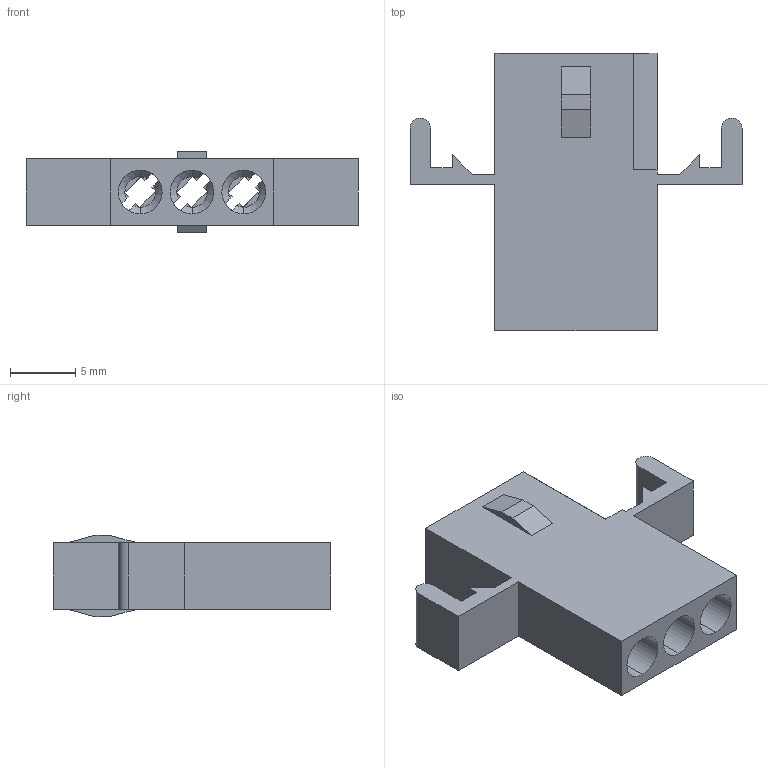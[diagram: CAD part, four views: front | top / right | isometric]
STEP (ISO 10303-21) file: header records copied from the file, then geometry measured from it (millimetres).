
FILE_DESCRIPTION (( 'STEP AP203' ), '1' );
FILE_NAME ('556-003-000-102.STEP', '2020-03-13T14:18:30', ( '' ), ( '' ), 'SwSTEP 2.0', 'SolidWorks 2016', '' );
FILE_SCHEMA (( 'CONFIG_CONTROL_DESIGN' ));
Length unit declared in the file: millimetre
Products named in the file (2): 556-003-000-102; 556-210-001_556-003-000-102
Assembly tree (1 placements, depth 2):
  556-003-000-102
    556-210-001_556-003-000-102
Bounding box: 25.4 x 21.21 x 6.22 mm (x, y, z)
Volume: 992.5 mm3; surface area: 1830.1 mm2
Topology: 1 solids, 1 shells, 116 faces, 330 edges, 218 vertices
Faces by surface type: plane 90, cylinder 20, cone 6
Entity records: 3994 total; most frequent: CARTESIAN_POINT 776, ORIENTED_EDGE 660, DIRECTION 598, EDGE_CURVE 330, LINE 230, VECTOR 230, VERTEX_POINT 218, AXIS2_PLACEMENT_3D 184
